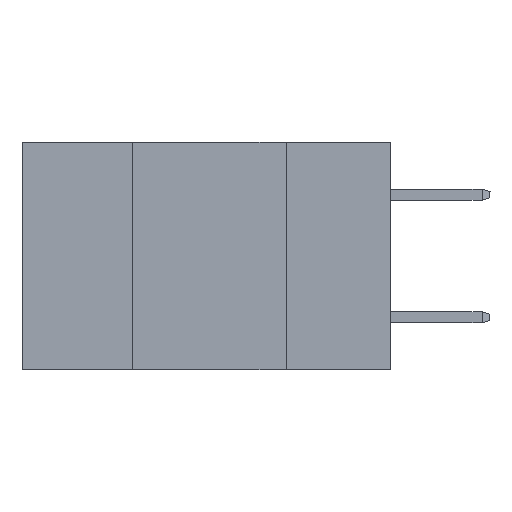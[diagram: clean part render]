
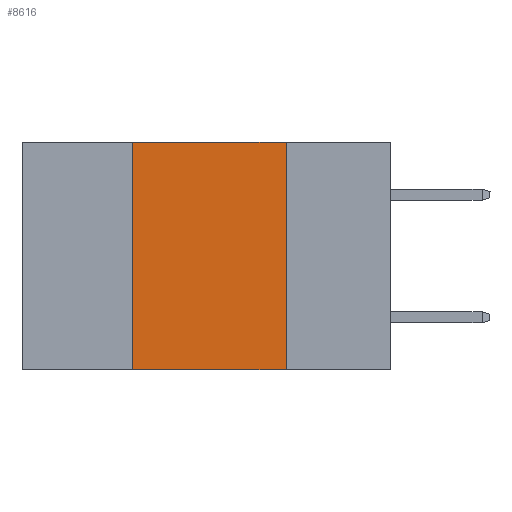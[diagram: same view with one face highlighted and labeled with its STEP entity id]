
A CAD part, left-side view. The second image highlights one B-rep face of the part: STEP entity #8616.
In plain terms, the highlighted planar face has unit normal (-1, 0, 0).
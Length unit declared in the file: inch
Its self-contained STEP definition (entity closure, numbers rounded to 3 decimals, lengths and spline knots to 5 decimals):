
#839 = CARTESIAN_POINT ( 'NONE',  ( 0., 0.42, -0.37 ) ) ;
#1396 = LINE ( 'NONE', #9503, #15273 ) ;
#2845 = DIRECTION ( 'NONE',  ( 1., 0., 0. ) ) ;
#3626 = VERTEX_POINT ( 'NONE', #839 ) ;
#4426 = ORIENTED_EDGE ( 'NONE', *, *, #15680, .F. ) ;
#4800 = AXIS2_PLACEMENT_3D ( 'NONE', #13676, #2845, #15471 ) ;
#4811 = LINE ( 'NONE', #12519, #23281 ) ;
#5004 = ORIENTED_EDGE ( 'NONE', *, *, #9705, .F. ) ;
#6111 = EDGE_LOOP ( 'NONE', ( #13478, #4426, #5004, #9861 ) ) ;
#6280 = CARTESIAN_POINT ( 'NONE',  ( 0., 0.6, -0.37 ) ) ;
#6333 = CARTESIAN_POINT ( 'NONE',  ( 0., 0.17, 0. ) ) ;
#6783 = EDGE_CURVE ( 'NONE', #3626, #21192, #14216, .T. ) ;
#7174 = DIRECTION ( 'NONE',  ( 0., 0., -1. ) ) ;
#7679 = CARTESIAN_POINT ( 'NONE',  ( 0., 0.17, -0.37 ) ) ;
#8616 = ADVANCED_FACE ( 'NONE', ( #9392 ), #22515, .F. ) ;
#8812 = EDGE_CURVE ( 'NONE', #9239, #21192, #4811, .T. ) ;
#9239 = VERTEX_POINT ( 'NONE', #6333 ) ;
#9392 = FACE_OUTER_BOUND ( 'NONE', #6111, .T. ) ;
#9482 = VECTOR ( 'NONE', #11825, 39.37008 ) ;
#9503 = CARTESIAN_POINT ( 'NONE',  ( 0., 0.42, 0. ) ) ;
#9705 = EDGE_CURVE ( 'NONE', #3626, #22876, #1396, .T. ) ;
#9861 = ORIENTED_EDGE ( 'NONE', *, *, #6783, .T. ) ;
#11312 = DIRECTION ( 'NONE',  ( 0., 0., 1. ) ) ;
#11531 = VECTOR ( 'NONE', #14735, 39.37008 ) ;
#11825 = DIRECTION ( 'NONE',  ( 0., -1., 0. ) ) ;
#12519 = CARTESIAN_POINT ( 'NONE',  ( 0., 0.17, 0. ) ) ;
#13478 = ORIENTED_EDGE ( 'NONE', *, *, #8812, .F. ) ;
#13676 = CARTESIAN_POINT ( 'NONE',  ( 0., 0.6, 0. ) ) ;
#14216 = LINE ( 'NONE', #6280, #9482 ) ;
#14735 = DIRECTION ( 'NONE',  ( 0., -1., 0. ) ) ;
#15273 = VECTOR ( 'NONE', #11312, 39.37008 ) ;
#15471 = DIRECTION ( 'NONE',  ( 0., 0., -1. ) ) ;
#15680 = EDGE_CURVE ( 'NONE', #22876, #9239, #16253, .T. ) ;
#16253 = LINE ( 'NONE', #21780, #11531 ) ;
#21075 = CARTESIAN_POINT ( 'NONE',  ( 0., 0.42, 0. ) ) ;
#21192 = VERTEX_POINT ( 'NONE', #7679 ) ;
#21780 = CARTESIAN_POINT ( 'NONE',  ( 0., 0.6, 0. ) ) ;
#22515 = PLANE ( 'NONE',  #4800 ) ;
#22876 = VERTEX_POINT ( 'NONE', #21075 ) ;
#23281 = VECTOR ( 'NONE', #7174, 39.37008 ) ;
